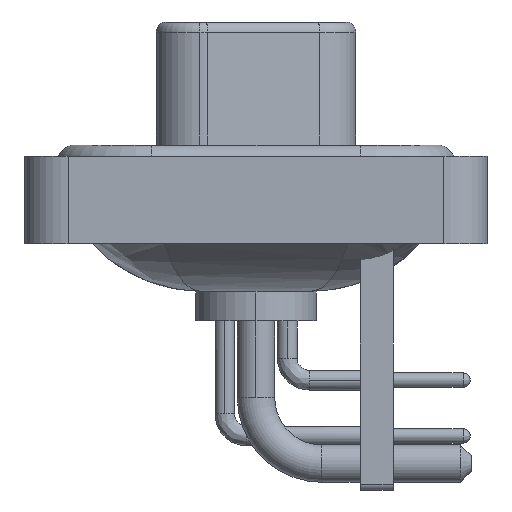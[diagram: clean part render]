
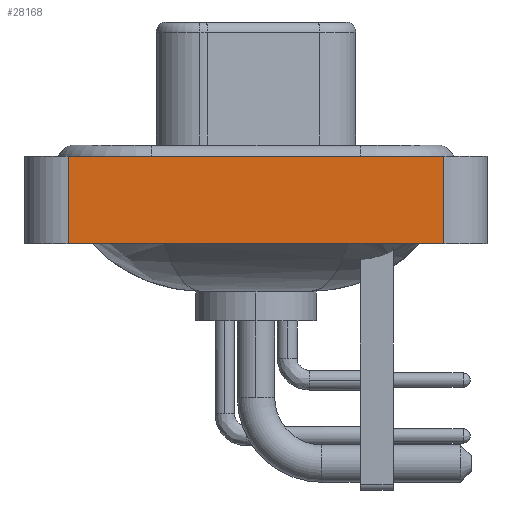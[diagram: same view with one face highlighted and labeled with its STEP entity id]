
A CAD part, left-side view. The second image highlights one B-rep face of the part: STEP entity #28168.
In plain terms, the highlighted planar face has unit normal (-1, 0, 0).
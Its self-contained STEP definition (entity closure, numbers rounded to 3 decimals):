
#1277 = CARTESIAN_POINT ( 'NONE',  ( -7.35, -8.55, -3.6 ) ) ;
#1551 = LINE ( 'NONE', #4226, #15580 ) ;
#1999 = DIRECTION ( 'NONE',  ( 0., -1., 0. ) ) ;
#2094 = EDGE_LOOP ( 'NONE', ( #26543, #18796, #26891, #7281 ) ) ;
#3311 = VERTEX_POINT ( 'NONE', #7291 ) ;
#3501 = LINE ( 'NONE', #1277, #19355 ) ;
#4181 = CARTESIAN_POINT ( 'NONE',  ( -7.35, -8.55, -3.6 ) ) ;
#4226 = CARTESIAN_POINT ( 'NONE',  ( -7.35, 8.55, -3.6 ) ) ;
#4804 = LINE ( 'NONE', #20163, #18180 ) ;
#6414 = EDGE_CURVE ( 'NONE', #29090, #10836, #4804, .T. ) ;
#7281 = ORIENTED_EDGE ( 'NONE', *, *, #11894, .T. ) ;
#7291 = CARTESIAN_POINT ( 'NONE',  ( -7.35, 8.55, -3.6 ) ) ;
#7647 = LINE ( 'NONE', #7934, #24614 ) ;
#7934 = CARTESIAN_POINT ( 'NONE',  ( -7.35, -8.55, 0.4 ) ) ;
#8694 = CARTESIAN_POINT ( 'NONE',  ( -7.35, -8.55, -3.6 ) ) ;
#10836 = VERTEX_POINT ( 'NONE', #19275 ) ;
#11101 = DIRECTION ( 'NONE',  ( -1., 0., 0. ) ) ;
#11894 = EDGE_CURVE ( 'NONE', #3311, #29090, #3501, .T. ) ;
#13806 = DIRECTION ( 'NONE',  ( 0., 0., 1. ) ) ;
#15580 = VECTOR ( 'NONE', #26228, 1000. ) ;
#15960 = PLANE ( 'NONE',  #24666 ) ;
#18180 = VECTOR ( 'NONE', #13806, 1000. ) ;
#18796 = ORIENTED_EDGE ( 'NONE', *, *, #21018, .F. ) ;
#19275 = CARTESIAN_POINT ( 'NONE',  ( -7.35, -8.55, 0.4 ) ) ;
#19355 = VECTOR ( 'NONE', #28306, 1000. ) ;
#20163 = CARTESIAN_POINT ( 'NONE',  ( -7.35, -8.55, -3.6 ) ) ;
#20677 = EDGE_CURVE ( 'NONE', #3311, #27527, #1551, .T. ) ;
#21018 = EDGE_CURVE ( 'NONE', #27527, #10836, #7647, .T. ) ;
#24564 = FACE_OUTER_BOUND ( 'NONE', #2094, .T. ) ;
#24614 = VECTOR ( 'NONE', #1999, 1000. ) ;
#24666 = AXIS2_PLACEMENT_3D ( 'NONE', #4181, #11101, #24996 ) ;
#24996 = DIRECTION ( 'NONE',  ( 0., 0., 1. ) ) ;
#26228 = DIRECTION ( 'NONE',  ( 0., 0., 1. ) ) ;
#26543 = ORIENTED_EDGE ( 'NONE', *, *, #6414, .T. ) ;
#26891 = ORIENTED_EDGE ( 'NONE', *, *, #20677, .F. ) ;
#27527 = VERTEX_POINT ( 'NONE', #28668 ) ;
#28168 = ADVANCED_FACE ( 'NONE', ( #24564 ), #15960, .T. ) ;
#28306 = DIRECTION ( 'NONE',  ( 0., -1., 0. ) ) ;
#28668 = CARTESIAN_POINT ( 'NONE',  ( -7.35, 8.55, 0.4 ) ) ;
#29090 = VERTEX_POINT ( 'NONE', #8694 ) ;
